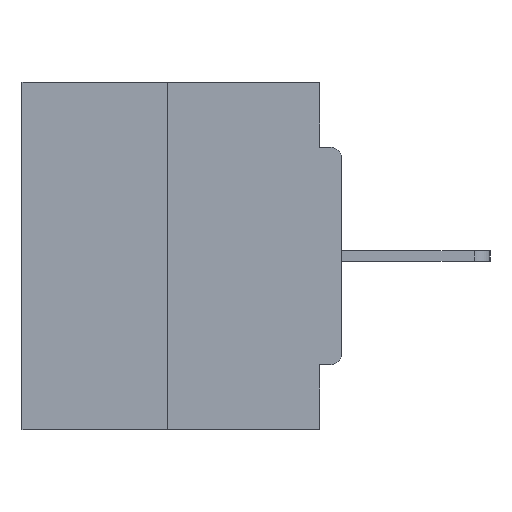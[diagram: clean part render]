
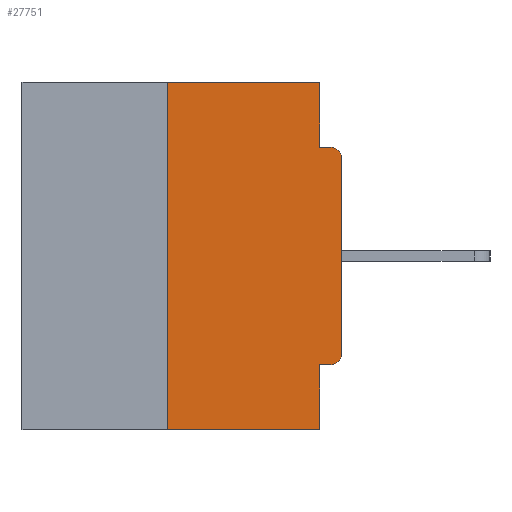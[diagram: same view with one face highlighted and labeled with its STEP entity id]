
A CAD part, left-side view. The second image highlights one B-rep face of the part: STEP entity #27751.
In plain terms, the highlighted planar face has unit normal (-1, 0, 0).
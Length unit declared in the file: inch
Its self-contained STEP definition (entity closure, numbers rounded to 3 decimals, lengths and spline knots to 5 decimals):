
#816 = CARTESIAN_POINT ( 'NONE',  ( 0., 0.031, 0. ) ) ;
#1018 = CARTESIAN_POINT ( 'NONE',  ( 0., 0.015, -0.3915 ) ) ;
#1062 = VERTEX_POINT ( 'NONE', #13700 ) ;
#1483 = DIRECTION ( 'NONE',  ( 0., 0., 1. ) ) ;
#1901 = ORIENTED_EDGE ( 'NONE', *, *, #3520, .F. ) ;
#2207 = DIRECTION ( 'NONE',  ( 0., 0., 1. ) ) ;
#2255 = EDGE_CURVE ( 'NONE', #29200, #13487, #13725, .T. ) ;
#3474 = LINE ( 'NONE', #8082, #34957 ) ;
#3520 = EDGE_CURVE ( 'NONE', #35950, #1062, #3474, .T. ) ;
#3563 = CARTESIAN_POINT ( 'NONE',  ( 0., 0.25, -0.5 ) ) ;
#4181 = EDGE_CURVE ( 'NONE', #21097, #29200, #11266, .T. ) ;
#6898 = VECTOR ( 'NONE', #38870, 39.37008 ) ;
#7737 = LINE ( 'NONE', #32011, #38041 ) ;
#7940 = DIRECTION ( 'NONE',  ( 0., 0., -1. ) ) ;
#8082 = CARTESIAN_POINT ( 'NONE',  ( 0., 0.46, 0. ) ) ;
#8107 = DIRECTION ( 'NONE',  ( -1., 0., 0. ) ) ;
#8225 = DIRECTION ( 'NONE',  ( -1., 0., 0. ) ) ;
#8306 = ORIENTED_EDGE ( 'NONE', *, *, #27674, .F. ) ;
#8641 = VERTEX_POINT ( 'NONE', #36923 ) ;
#9166 = EDGE_CURVE ( 'NONE', #21868, #19204, #14515, .T. ) ;
#11266 = CIRCLE ( 'NONE', #13387, 0.015 ) ;
#12082 = CARTESIAN_POINT ( 'NONE',  ( 0., 0.031, -0.4065 ) ) ;
#12123 = CARTESIAN_POINT ( 'NONE',  ( 0., 0.46, 0. ) ) ;
#12192 = ORIENTED_EDGE ( 'NONE', *, *, #19011, .T. ) ;
#12636 = ORIENTED_EDGE ( 'NONE', *, *, #27530, .F. ) ;
#13288 = VECTOR ( 'NONE', #25406, 39.37008 ) ;
#13387 = AXIS2_PLACEMENT_3D ( 'NONE', #1018, #8225, #7940 ) ;
#13487 = VERTEX_POINT ( 'NONE', #17479 ) ;
#13700 = CARTESIAN_POINT ( 'NONE',  ( 0., 0.031, 0. ) ) ;
#13725 = LINE ( 'NONE', #38406, #14697 ) ;
#14509 = AXIS2_PLACEMENT_3D ( 'NONE', #12123, #36236, #18203 ) ;
#14515 = LINE ( 'NONE', #24251, #21558 ) ;
#14697 = VECTOR ( 'NONE', #2207, 39.37008 ) ;
#15175 = PLANE ( 'NONE',  #14509 ) ;
#16383 = CIRCLE ( 'NONE', #35753, 0.015 ) ;
#16407 = VERTEX_POINT ( 'NONE', #12082 ) ;
#16936 = ORIENTED_EDGE ( 'NONE', *, *, #27912, .F. ) ;
#17479 = CARTESIAN_POINT ( 'NONE',  ( 0., 0., -0.1085 ) ) ;
#18203 = DIRECTION ( 'NONE',  ( 0., 0., -1. ) ) ;
#19011 = EDGE_CURVE ( 'NONE', #13487, #32333, #16383, .T. ) ;
#19204 = VERTEX_POINT ( 'NONE', #27234 ) ;
#19848 = VECTOR ( 'NONE', #23232, 39.37008 ) ;
#20125 = DIRECTION ( 'NONE',  ( 0., -1., 0. ) ) ;
#21097 = VERTEX_POINT ( 'NONE', #32976 ) ;
#21558 = VECTOR ( 'NONE', #27292, 39.37008 ) ;
#21868 = VERTEX_POINT ( 'NONE', #3563 ) ;
#21997 = DIRECTION ( 'NONE',  ( 0., -1., 0. ) ) ;
#22642 = LINE ( 'NONE', #27984, #37727 ) ;
#23232 = DIRECTION ( 'NONE',  ( 0., 0., -1. ) ) ;
#23952 = CARTESIAN_POINT ( 'NONE',  ( 0., 0.25, 0. ) ) ;
#24251 = CARTESIAN_POINT ( 'NONE',  ( 0., 0.46, -0.5 ) ) ;
#25406 = DIRECTION ( 'NONE',  ( 0., 0., -1. ) ) ;
#25428 = ORIENTED_EDGE ( 'NONE', *, *, #4181, .T. ) ;
#26315 = CARTESIAN_POINT ( 'NONE',  ( 0., 0.015, -0.1085 ) ) ;
#26845 = EDGE_CURVE ( 'NONE', #1062, #8641, #29376, .T. ) ;
#27234 = CARTESIAN_POINT ( 'NONE',  ( 0., 0.031, -0.5 ) ) ;
#27292 = DIRECTION ( 'NONE',  ( 0., -1., 0. ) ) ;
#27530 = EDGE_CURVE ( 'NONE', #16407, #19204, #28851, .T. ) ;
#27674 = EDGE_CURVE ( 'NONE', #21097, #16407, #31207, .T. ) ;
#27751 = ADVANCED_FACE ( 'NONE', ( #35405 ), #15175, .F. ) ;
#27912 = EDGE_CURVE ( 'NONE', #8641, #32333, #22642, .T. ) ;
#27984 = CARTESIAN_POINT ( 'NONE',  ( 0., 0., -0.0935 ) ) ;
#28747 = CARTESIAN_POINT ( 'NONE',  ( 0., 0.015, -0.0935 ) ) ;
#28851 = LINE ( 'NONE', #38215, #19848 ) ;
#29200 = VERTEX_POINT ( 'NONE', #32876 ) ;
#29240 = ORIENTED_EDGE ( 'NONE', *, *, #9166, .T. ) ;
#29362 = DIRECTION ( 'NONE',  ( 0., 0., -1. ) ) ;
#29376 = LINE ( 'NONE', #816, #13288 ) ;
#31207 = LINE ( 'NONE', #32893, #6898 ) ;
#32011 = CARTESIAN_POINT ( 'NONE',  ( 0., 0.25, 0. ) ) ;
#32333 = VERTEX_POINT ( 'NONE', #28747 ) ;
#32876 = CARTESIAN_POINT ( 'NONE',  ( 0., 0., -0.3915 ) ) ;
#32893 = CARTESIAN_POINT ( 'NONE',  ( 0., 0., -0.4065 ) ) ;
#32976 = CARTESIAN_POINT ( 'NONE',  ( 0., 0.015, -0.4065 ) ) ;
#32986 = EDGE_CURVE ( 'NONE', #21868, #35950, #7737, .T. ) ;
#34899 = ORIENTED_EDGE ( 'NONE', *, *, #26845, .F. ) ;
#34957 = VECTOR ( 'NONE', #20125, 39.37008 ) ;
#35331 = ORIENTED_EDGE ( 'NONE', *, *, #2255, .T. ) ;
#35405 = FACE_OUTER_BOUND ( 'NONE', #39074, .T. ) ;
#35753 = AXIS2_PLACEMENT_3D ( 'NONE', #26315, #8107, #29362 ) ;
#35950 = VERTEX_POINT ( 'NONE', #23952 ) ;
#36236 = DIRECTION ( 'NONE',  ( 1., 0., 0. ) ) ;
#36247 = ORIENTED_EDGE ( 'NONE', *, *, #32986, .F. ) ;
#36923 = CARTESIAN_POINT ( 'NONE',  ( 0., 0.031, -0.0935 ) ) ;
#37727 = VECTOR ( 'NONE', #21997, 39.37008 ) ;
#38041 = VECTOR ( 'NONE', #1483, 39.37008 ) ;
#38215 = CARTESIAN_POINT ( 'NONE',  ( 0., 0.031, -0.5 ) ) ;
#38406 = CARTESIAN_POINT ( 'NONE',  ( 0., 0., 0. ) ) ;
#38870 = DIRECTION ( 'NONE',  ( 0., 1., 0. ) ) ;
#39074 = EDGE_LOOP ( 'NONE', ( #1901, #36247, #29240, #12636, #8306, #25428, #35331, #12192, #16936, #34899 ) ) ;
